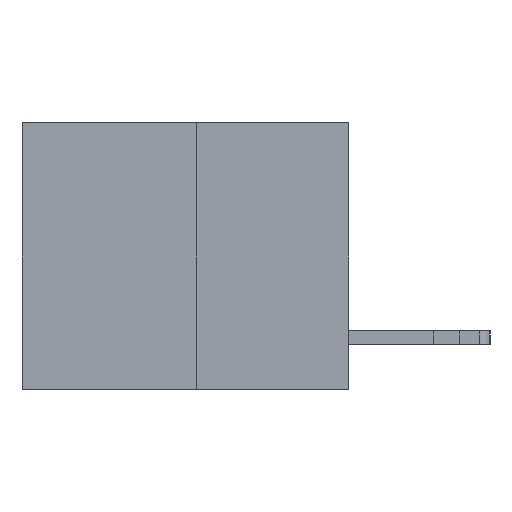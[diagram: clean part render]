
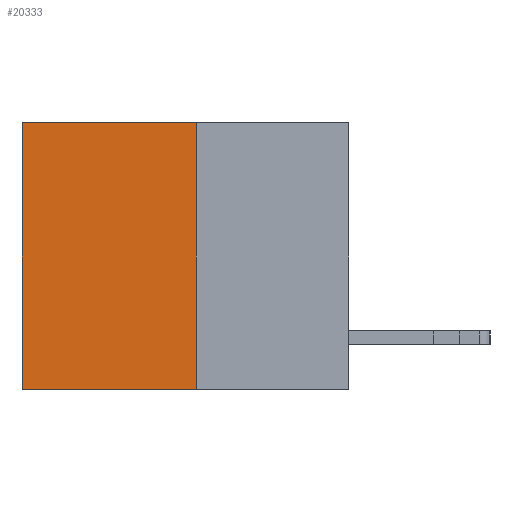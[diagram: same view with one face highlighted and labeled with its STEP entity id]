
A CAD part, left-side view. The second image highlights one B-rep face of the part: STEP entity #20333.
In plain terms, the highlighted planar face has unit normal (-1, 0, 0).
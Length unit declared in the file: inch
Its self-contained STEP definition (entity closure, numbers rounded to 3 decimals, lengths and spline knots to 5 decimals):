
#286 = VERTEX_POINT ( 'NONE', #10411 ) ;
#568 = DIRECTION ( 'NONE',  ( 1., 0., 0. ) ) ;
#1608 = CARTESIAN_POINT ( 'NONE',  ( 0.3165, 0.28, -0.49 ) ) ;
#1737 = LINE ( 'NONE', #12590, #13866 ) ;
#1772 = ORIENTED_EDGE ( 'NONE', *, *, #14789, .T. ) ;
#2463 = DIRECTION ( 'NONE',  ( 0., 0., -1. ) ) ;
#3001 = CARTESIAN_POINT ( 'NONE',  ( 0.3165, 0.6, -0.49 ) ) ;
#4049 = VERTEX_POINT ( 'NONE', #8242 ) ;
#6556 = EDGE_CURVE ( 'NONE', #286, #8330, #17699, .T. ) ;
#7261 = VECTOR ( 'NONE', #7499, 39.37008 ) ;
#7499 = DIRECTION ( 'NONE',  ( 0., 0., -1. ) ) ;
#8242 = CARTESIAN_POINT ( 'NONE',  ( 0.3165, 0.28, 0. ) ) ;
#8330 = VERTEX_POINT ( 'NONE', #3001 ) ;
#8966 = DIRECTION ( 'NONE',  ( 0., 1., 0. ) ) ;
#10157 = VERTEX_POINT ( 'NONE', #25007 ) ;
#10328 = LINE ( 'NONE', #16687, #24329 ) ;
#10411 = CARTESIAN_POINT ( 'NONE',  ( 0.3165, 0.28, -0.49 ) ) ;
#12526 = VECTOR ( 'NONE', #15658, 39.37008 ) ;
#12590 = CARTESIAN_POINT ( 'NONE',  ( 0.3165, 0.6, -0.49 ) ) ;
#13866 = VECTOR ( 'NONE', #18117, 39.37008 ) ;
#13923 = ORIENTED_EDGE ( 'NONE', *, *, #6556, .F. ) ;
#14789 = EDGE_CURVE ( 'NONE', #4049, #10157, #10328, .T. ) ;
#15309 = CARTESIAN_POINT ( 'NONE',  ( 0.3165, 0.28, -0.49 ) ) ;
#15658 = DIRECTION ( 'NONE',  ( 0., 1., 0. ) ) ;
#16096 = LINE ( 'NONE', #15309, #7261 ) ;
#16687 = CARTESIAN_POINT ( 'NONE',  ( 0.3165, 0.28, 0. ) ) ;
#17454 = EDGE_CURVE ( 'NONE', #4049, #286, #16096, .T. ) ;
#17699 = LINE ( 'NONE', #1608, #12526 ) ;
#17992 = PLANE ( 'NONE',  #18129 ) ;
#18117 = DIRECTION ( 'NONE',  ( 0., 0., -1. ) ) ;
#18129 = AXIS2_PLACEMENT_3D ( 'NONE', #18310, #568, #2463 ) ;
#18310 = CARTESIAN_POINT ( 'NONE',  ( 0.3165, 0.28, -0.49 ) ) ;
#19312 = EDGE_LOOP ( 'NONE', ( #24169, #13923, #20974, #1772 ) ) ;
#20333 = ADVANCED_FACE ( 'NONE', ( #20793 ), #17992, .F. ) ;
#20793 = FACE_OUTER_BOUND ( 'NONE', #19312, .T. ) ;
#20974 = ORIENTED_EDGE ( 'NONE', *, *, #17454, .F. ) ;
#21013 = EDGE_CURVE ( 'NONE', #10157, #8330, #1737, .T. ) ;
#24169 = ORIENTED_EDGE ( 'NONE', *, *, #21013, .T. ) ;
#24329 = VECTOR ( 'NONE', #8966, 39.37008 ) ;
#25007 = CARTESIAN_POINT ( 'NONE',  ( 0.3165, 0.6, 0. ) ) ;
